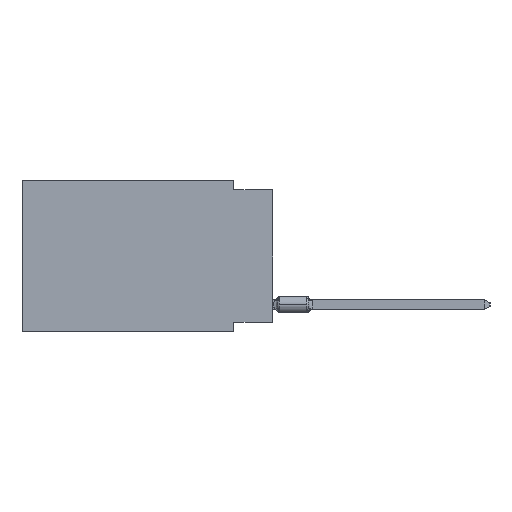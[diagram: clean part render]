
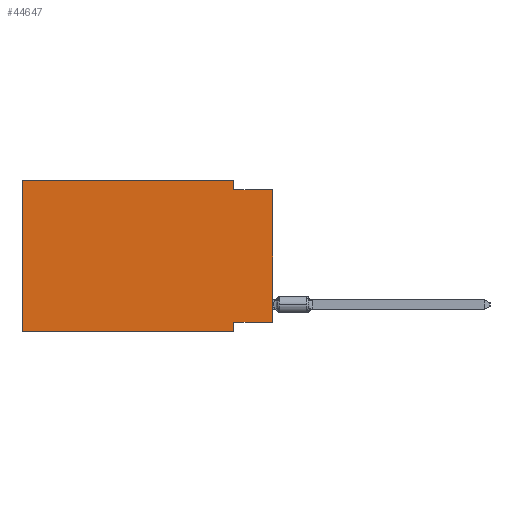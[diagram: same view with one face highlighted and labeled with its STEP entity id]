
A CAD part, left-side view. The second image highlights one B-rep face of the part: STEP entity #44647.
In plain terms, the highlighted planar face has unit normal (-1, 0, 0).
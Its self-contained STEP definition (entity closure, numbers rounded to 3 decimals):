
#75 = LINE ( 'NONE', #26013, #1110 ) ;
#650 = EDGE_CURVE ( 'NONE', #31557, #6048, #75, .T. ) ;
#1110 = VECTOR ( 'NONE', #54395, 1000. ) ;
#1410 = PLANE ( 'NONE',  #27259 ) ;
#2781 = VECTOR ( 'NONE', #3762, 1000. ) ;
#3199 = VERTEX_POINT ( 'NONE', #22739 ) ;
#3320 = ORIENTED_EDGE ( 'NONE', *, *, #56717, .F. ) ;
#3762 = DIRECTION ( 'NONE',  ( 0., -1., 0. ) ) ;
#4150 = CARTESIAN_POINT ( 'NONE',  ( 0., 0., 0. ) ) ;
#4529 = EDGE_CURVE ( 'NONE', #79179, #37006, #57240, .T. ) ;
#6048 = VERTEX_POINT ( 'NONE', #15975 ) ;
#9857 = CARTESIAN_POINT ( 'NONE',  ( 0., 0., -0.635 ) ) ;
#10773 = LINE ( 'NONE', #62196, #67520 ) ;
#12047 = VECTOR ( 'NONE', #63145, 1000. ) ;
#14092 = EDGE_LOOP ( 'NONE', ( #63021, #30097, #71548, #34345, #52359, #23423, #3320, #76067 ) ) ;
#15975 = CARTESIAN_POINT ( 'NONE',  ( 0., 16.383, 0. ) ) ;
#16437 = VECTOR ( 'NONE', #62117, 1000. ) ;
#17860 = EDGE_CURVE ( 'NONE', #31557, #23301, #30118, .T. ) ;
#22739 = CARTESIAN_POINT ( 'NONE',  ( 0., 2.54, -9.271 ) ) ;
#23121 = CARTESIAN_POINT ( 'NONE',  ( 0., 0., -0.635 ) ) ;
#23301 = VERTEX_POINT ( 'NONE', #30063 ) ;
#23423 = ORIENTED_EDGE ( 'NONE', *, *, #17860, .T. ) ;
#24910 = LINE ( 'NONE', #62723, #12047 ) ;
#26013 = CARTESIAN_POINT ( 'NONE',  ( 0., 16.383, 0. ) ) ;
#27259 = AXIS2_PLACEMENT_3D ( 'NONE', #28590, #72358, #34978 ) ;
#27529 = VECTOR ( 'NONE', #72295, 1000. ) ;
#28590 = CARTESIAN_POINT ( 'NONE',  ( 0., 16.383, 0. ) ) ;
#29833 = CARTESIAN_POINT ( 'NONE',  ( 0., 16.383, 0. ) ) ;
#30063 = CARTESIAN_POINT ( 'NONE',  ( 0., 2.54, -9.906 ) ) ;
#30097 = ORIENTED_EDGE ( 'NONE', *, *, #38756, .F. ) ;
#30118 = LINE ( 'NONE', #61978, #2781 ) ;
#31557 = VERTEX_POINT ( 'NONE', #76857 ) ;
#31774 = CARTESIAN_POINT ( 'NONE',  ( 0., 2.54, 0. ) ) ;
#33109 = VERTEX_POINT ( 'NONE', #57228 ) ;
#34345 = ORIENTED_EDGE ( 'NONE', *, *, #54287, .F. ) ;
#34978 = DIRECTION ( 'NONE',  ( 0., 0., -1. ) ) ;
#35857 = DIRECTION ( 'NONE',  ( 0., -1., 0. ) ) ;
#37006 = VERTEX_POINT ( 'NONE', #9857 ) ;
#37035 = LINE ( 'NONE', #29833, #16437 ) ;
#38756 = EDGE_CURVE ( 'NONE', #33109, #37006, #41806, .T. ) ;
#40993 = EDGE_CURVE ( 'NONE', #64674, #33109, #10773, .T. ) ;
#41806 = LINE ( 'NONE', #23121, #67469 ) ;
#42382 = DIRECTION ( 'NONE',  ( 0., 0., 1. ) ) ;
#44647 = ADVANCED_FACE ( 'NONE', ( #46437 ), #1410, .F. ) ;
#46437 = FACE_OUTER_BOUND ( 'NONE', #14092, .T. ) ;
#47228 = CARTESIAN_POINT ( 'NONE',  ( 0., 2.54, -9.906 ) ) ;
#50260 = DIRECTION ( 'NONE',  ( 0., 0., -1. ) ) ;
#51857 = VECTOR ( 'NONE', #42382, 1000. ) ;
#52359 = ORIENTED_EDGE ( 'NONE', *, *, #650, .F. ) ;
#54287 = EDGE_CURVE ( 'NONE', #6048, #64674, #37035, .T. ) ;
#54395 = DIRECTION ( 'NONE',  ( 0., 0., 1. ) ) ;
#56717 = EDGE_CURVE ( 'NONE', #3199, #23301, #67187, .T. ) ;
#57228 = CARTESIAN_POINT ( 'NONE',  ( 0., 2.54, -0.635 ) ) ;
#57240 = LINE ( 'NONE', #4150, #51857 ) ;
#61978 = CARTESIAN_POINT ( 'NONE',  ( 0., 16.383, -9.906 ) ) ;
#62117 = DIRECTION ( 'NONE',  ( 0., -1., 0. ) ) ;
#62196 = CARTESIAN_POINT ( 'NONE',  ( 0., 2.54, 0. ) ) ;
#62723 = CARTESIAN_POINT ( 'NONE',  ( 0., 0., -9.271 ) ) ;
#63021 = ORIENTED_EDGE ( 'NONE', *, *, #4529, .T. ) ;
#63145 = DIRECTION ( 'NONE',  ( 0., 1., 0. ) ) ;
#64674 = VERTEX_POINT ( 'NONE', #31774 ) ;
#66093 = EDGE_CURVE ( 'NONE', #79179, #3199, #24910, .T. ) ;
#67187 = LINE ( 'NONE', #47228, #27529 ) ;
#67469 = VECTOR ( 'NONE', #35857, 1000. ) ;
#67520 = VECTOR ( 'NONE', #50260, 1000. ) ;
#69239 = CARTESIAN_POINT ( 'NONE',  ( 0., 0., -9.271 ) ) ;
#71548 = ORIENTED_EDGE ( 'NONE', *, *, #40993, .F. ) ;
#72295 = DIRECTION ( 'NONE',  ( 0., 0., -1. ) ) ;
#72358 = DIRECTION ( 'NONE',  ( 1., 0., 0. ) ) ;
#76067 = ORIENTED_EDGE ( 'NONE', *, *, #66093, .F. ) ;
#76857 = CARTESIAN_POINT ( 'NONE',  ( 0., 16.383, -9.906 ) ) ;
#79179 = VERTEX_POINT ( 'NONE', #69239 ) ;
